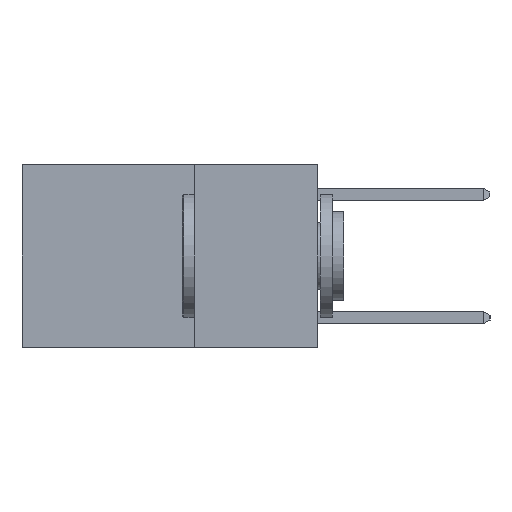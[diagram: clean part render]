
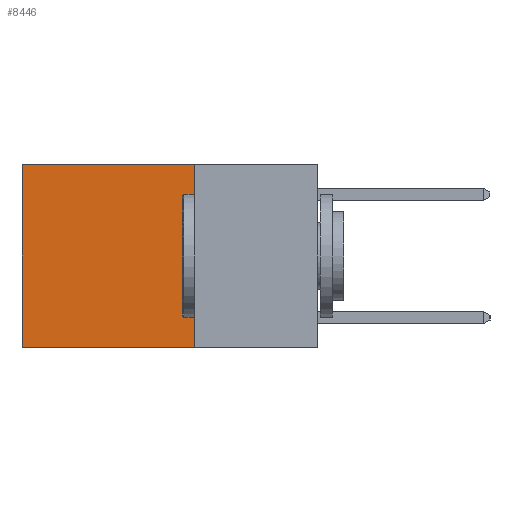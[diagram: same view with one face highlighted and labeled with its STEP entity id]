
A CAD part, left-side view. The second image highlights one B-rep face of the part: STEP entity #8446.
In plain terms, the highlighted planar face has unit normal (-1, 0, 0).
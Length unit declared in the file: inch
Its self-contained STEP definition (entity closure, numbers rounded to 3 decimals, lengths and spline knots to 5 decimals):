
#57 = LINE ( 'NONE', #843, #7247 ) ;
#538 = AXIS2_PLACEMENT_3D ( 'NONE', #8517, #1327, #6444 ) ;
#571 = DIRECTION ( 'NONE',  ( 0., 0., -1. ) ) ;
#653 = VECTOR ( 'NONE', #571, 39.37008 ) ;
#838 = CARTESIAN_POINT ( 'NONE',  ( 0.2625, 0.6, -0.37 ) ) ;
#843 = CARTESIAN_POINT ( 'NONE',  ( 0.2625, 0.6, 0. ) ) ;
#1246 = VERTEX_POINT ( 'NONE', #2563 ) ;
#1327 = DIRECTION ( 'NONE',  ( 1., 0., 0. ) ) ;
#1968 = CARTESIAN_POINT ( 'NONE',  ( 0.2625, 0.25, 0. ) ) ;
#2108 = CARTESIAN_POINT ( 'NONE',  ( 0.2625, 0.25, -0.37 ) ) ;
#2306 = DIRECTION ( 'NONE',  ( 0., 0., -1. ) ) ;
#2376 = VECTOR ( 'NONE', #7755, 39.37008 ) ;
#2563 = CARTESIAN_POINT ( 'NONE',  ( 0.2625, 0.25, -0.37 ) ) ;
#2604 = DIRECTION ( 'NONE',  ( 0., 1., 0. ) ) ;
#2658 = FACE_OUTER_BOUND ( 'NONE', #7580, .T. ) ;
#2852 = EDGE_CURVE ( 'NONE', #1246, #5893, #5223, .T. ) ;
#3405 = CARTESIAN_POINT ( 'NONE',  ( 0.2625, 0.6, 0. ) ) ;
#3613 = EDGE_CURVE ( 'NONE', #6211, #1246, #4805, .T. ) ;
#3684 = CARTESIAN_POINT ( 'NONE',  ( 0.2625, 0.25, 0. ) ) ;
#3889 = EDGE_CURVE ( 'NONE', #6211, #5052, #7876, .T. ) ;
#4805 = LINE ( 'NONE', #8488, #653 ) ;
#5052 = VERTEX_POINT ( 'NONE', #3405 ) ;
#5223 = LINE ( 'NONE', #2108, #8732 ) ;
#5724 = PLANE ( 'NONE',  #538 ) ;
#5725 = ORIENTED_EDGE ( 'NONE', *, *, #3613, .F. ) ;
#5893 = VERTEX_POINT ( 'NONE', #838 ) ;
#6211 = VERTEX_POINT ( 'NONE', #1968 ) ;
#6444 = DIRECTION ( 'NONE',  ( 0., 0., -1. ) ) ;
#7247 = VECTOR ( 'NONE', #2306, 39.37008 ) ;
#7580 = EDGE_LOOP ( 'NONE', ( #9090, #8913, #5725, #8449 ) ) ;
#7755 = DIRECTION ( 'NONE',  ( 0., 1., 0. ) ) ;
#7876 = LINE ( 'NONE', #3684, #2376 ) ;
#7987 = EDGE_CURVE ( 'NONE', #5052, #5893, #57, .T. ) ;
#8446 = ADVANCED_FACE ( 'NONE', ( #2658 ), #5724, .F. ) ;
#8449 = ORIENTED_EDGE ( 'NONE', *, *, #3889, .T. ) ;
#8488 = CARTESIAN_POINT ( 'NONE',  ( 0.2625, 0.25, 0. ) ) ;
#8517 = CARTESIAN_POINT ( 'NONE',  ( 0.2625, 0.25, 0. ) ) ;
#8732 = VECTOR ( 'NONE', #2604, 39.37008 ) ;
#8913 = ORIENTED_EDGE ( 'NONE', *, *, #2852, .F. ) ;
#9090 = ORIENTED_EDGE ( 'NONE', *, *, #7987, .T. ) ;
